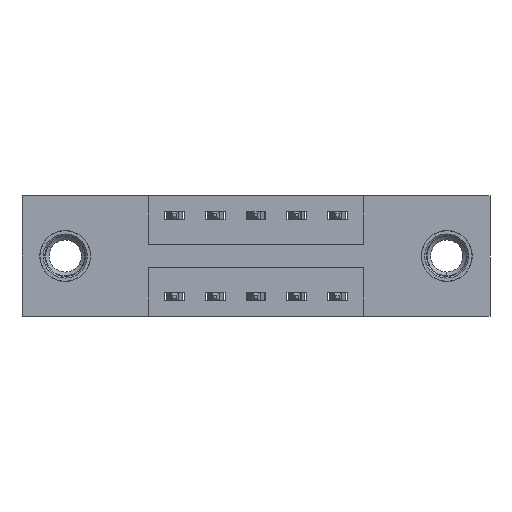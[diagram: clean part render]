
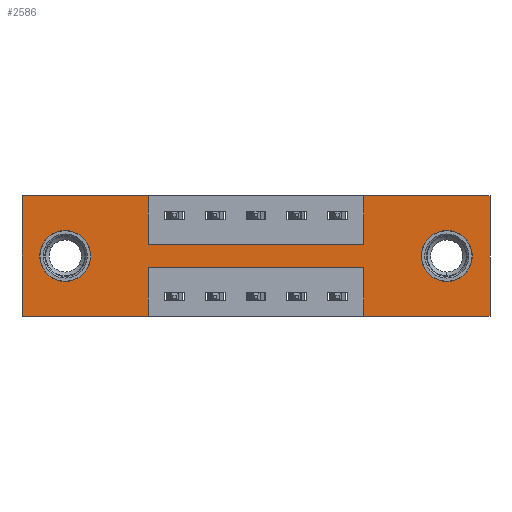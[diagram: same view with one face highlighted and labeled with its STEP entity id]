
A CAD part, front view. The second image highlights one B-rep face of the part: STEP entity #2586.
In plain terms, the highlighted planar face has unit normal (0, -1, 0).
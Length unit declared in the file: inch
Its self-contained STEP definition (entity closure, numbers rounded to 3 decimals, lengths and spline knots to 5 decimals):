
#34 = ORIENTED_EDGE ( 'NONE', *, *, #7145, .F. ) ;
#138 = CARTESIAN_POINT ( 'NONE',  ( 1.0475, 0., -0.37 ) ) ;
#144 = EDGE_CURVE ( 'NONE', #8442, #2010, #308, .T. ) ;
#201 = LINE ( 'NONE', #477, #5278 ) ;
#285 = AXIS2_PLACEMENT_3D ( 'NONE', #3052, #1589, #2337 ) ;
#308 = LINE ( 'NONE', #1299, #7852 ) ;
#352 = VECTOR ( 'NONE', #3183, 39.37008 ) ;
#371 = CARTESIAN_POINT ( 'NONE',  ( 1.0475, 0., 0. ) ) ;
#477 = CARTESIAN_POINT ( 'NONE',  ( 0.3875, 0., -0.22 ) ) ;
#523 = CARTESIAN_POINT ( 'NONE',  ( 0., 0., 0. ) ) ;
#541 = ORIENTED_EDGE ( 'NONE', *, *, #144, .F. ) ;
#603 = EDGE_CURVE ( 'NONE', #8182, #4735, #4690, .T. ) ;
#714 = EDGE_CURVE ( 'NONE', #3552, #2318, #6681, .T. ) ;
#733 = DIRECTION ( 'NONE',  ( 0., 1., 0. ) ) ;
#803 = CARTESIAN_POINT ( 'NONE',  ( 1.3025, 0., -0.185 ) ) ;
#824 = ORIENTED_EDGE ( 'NONE', *, *, #1951, .F. ) ;
#842 = ORIENTED_EDGE ( 'NONE', *, *, #8638, .F. ) ;
#930 = CARTESIAN_POINT ( 'NONE',  ( 0.1325, 0., -0.107 ) ) ;
#1009 = AXIS2_PLACEMENT_3D ( 'NONE', #3144, #6067, #7559 ) ;
#1018 = CARTESIAN_POINT ( 'NONE',  ( 1.3025, 0., -0.107 ) ) ;
#1029 = CARTESIAN_POINT ( 'NONE',  ( 0.3875, 0., -0.37 ) ) ;
#1113 = VECTOR ( 'NONE', #6441, 39.37008 ) ;
#1117 = ORIENTED_EDGE ( 'NONE', *, *, #6312, .F. ) ;
#1160 = VERTEX_POINT ( 'NONE', #3002 ) ;
#1279 = CARTESIAN_POINT ( 'NONE',  ( 0.3875, 0., 0. ) ) ;
#1299 = CARTESIAN_POINT ( 'NONE',  ( 0., 0., -0.37 ) ) ;
#1453 = CIRCLE ( 'NONE', #1009, 0.078 ) ;
#1497 = CARTESIAN_POINT ( 'NONE',  ( 0., 0., 0. ) ) ;
#1589 = DIRECTION ( 'NONE',  ( 0., -1., 0. ) ) ;
#1654 = ORIENTED_EDGE ( 'NONE', *, *, #3558, .F. ) ;
#1706 = EDGE_LOOP ( 'NONE', ( #4394, #842, #2827, #1654, #824, #2341, #4099, #1117, #34, #1812, #7414, #541 ) ) ;
#1734 = EDGE_CURVE ( 'NONE', #4735, #8182, #1453, .T. ) ;
#1739 = VERTEX_POINT ( 'NONE', #2428 ) ;
#1812 = ORIENTED_EDGE ( 'NONE', *, *, #714, .F. ) ;
#1835 = DIRECTION ( 'NONE',  ( 0., 0., -1. ) ) ;
#1866 = DIRECTION ( 'NONE',  ( 0., 0., 1. ) ) ;
#1901 = DIRECTION ( 'NONE',  ( 1., 0., 0. ) ) ;
#1946 = DIRECTION ( 'NONE',  ( 0., 0., 1. ) ) ;
#1951 = EDGE_CURVE ( 'NONE', #2083, #1739, #7568, .T. ) ;
#2010 = VERTEX_POINT ( 'NONE', #6331 ) ;
#2067 = CARTESIAN_POINT ( 'NONE',  ( 0.1325, 0., -0.185 ) ) ;
#2083 = VERTEX_POINT ( 'NONE', #2838 ) ;
#2204 = EDGE_LOOP ( 'NONE', ( #6551, #8420 ) ) ;
#2233 = LINE ( 'NONE', #1029, #7518 ) ;
#2293 = CARTESIAN_POINT ( 'NONE',  ( 0.3875, 0., -0.37 ) ) ;
#2318 = VERTEX_POINT ( 'NONE', #3682 ) ;
#2337 = DIRECTION ( 'NONE',  ( 0., 0., -1. ) ) ;
#2341 = ORIENTED_EDGE ( 'NONE', *, *, #3875, .F. ) ;
#2377 = LINE ( 'NONE', #4600, #352 ) ;
#2428 = CARTESIAN_POINT ( 'NONE',  ( 1.435, 0., -0.37 ) ) ;
#2482 = ORIENTED_EDGE ( 'NONE', *, *, #1734, .T. ) ;
#2554 = CARTESIAN_POINT ( 'NONE',  ( 0., 0., 0. ) ) ;
#2586 = ADVANCED_FACE ( 'NONE', ( #3332, #8987, #6343 ), #8069, .T. ) ;
#2632 = LINE ( 'NONE', #1497, #1113 ) ;
#2732 = VECTOR ( 'NONE', #4828, 39.37008 ) ;
#2827 = ORIENTED_EDGE ( 'NONE', *, *, #5557, .F. ) ;
#2838 = CARTESIAN_POINT ( 'NONE',  ( 1.435, 0., 0. ) ) ;
#2844 = DIRECTION ( 'NONE',  ( -1., 0., 0. ) ) ;
#3002 = CARTESIAN_POINT ( 'NONE',  ( 0.3875, 0., -0.15 ) ) ;
#3052 = CARTESIAN_POINT ( 'NONE',  ( 0., 0., -0.37 ) ) ;
#3058 = CARTESIAN_POINT ( 'NONE',  ( 1.0475, 0., -0.22 ) ) ;
#3084 = DIRECTION ( 'NONE',  ( -1., 0., 0. ) ) ;
#3144 = CARTESIAN_POINT ( 'NONE',  ( 1.3025, 0., -0.185 ) ) ;
#3183 = DIRECTION ( 'NONE',  ( 1., 0., 0. ) ) ;
#3316 = CARTESIAN_POINT ( 'NONE',  ( 0., 0., 0. ) ) ;
#3326 = AXIS2_PLACEMENT_3D ( 'NONE', #803, #733, #5906 ) ;
#3332 = FACE_BOUND ( 'NONE', #8821, .T. ) ;
#3365 = VECTOR ( 'NONE', #1946, 39.37008 ) ;
#3400 = EDGE_CURVE ( 'NONE', #2010, #3552, #3586, .T. ) ;
#3552 = VERTEX_POINT ( 'NONE', #523 ) ;
#3558 = EDGE_CURVE ( 'NONE', #1739, #6993, #7531, .T. ) ;
#3564 = DIRECTION ( 'NONE',  ( 0., 0., -1. ) ) ;
#3578 = CARTESIAN_POINT ( 'NONE',  ( 0.1325, 0., -0.263 ) ) ;
#3586 = LINE ( 'NONE', #3316, #3365 ) ;
#3637 = VERTEX_POINT ( 'NONE', #3725 ) ;
#3676 = DIRECTION ( 'NONE',  ( 0., 0., 1. ) ) ;
#3682 = CARTESIAN_POINT ( 'NONE',  ( 0.3875, 0., 0. ) ) ;
#3725 = CARTESIAN_POINT ( 'NONE',  ( 1.0475, 0., -0.15 ) ) ;
#3872 = VECTOR ( 'NONE', #1901, 39.37008 ) ;
#3875 = EDGE_CURVE ( 'NONE', #8345, #2083, #2632, .T. ) ;
#3980 = LINE ( 'NONE', #371, #8834 ) ;
#4028 = CARTESIAN_POINT ( 'NONE',  ( 1.435, 0., 0. ) ) ;
#4099 = ORIENTED_EDGE ( 'NONE', *, *, #4216, .F. ) ;
#4163 = CIRCLE ( 'NONE', #7188, 0.078 ) ;
#4216 = EDGE_CURVE ( 'NONE', #3637, #8345, #3980, .T. ) ;
#4343 = CIRCLE ( 'NONE', #4488, 0.078 ) ;
#4394 = ORIENTED_EDGE ( 'NONE', *, *, #9007, .F. ) ;
#4488 = AXIS2_PLACEMENT_3D ( 'NONE', #8062, #8000, #3676 ) ;
#4600 = CARTESIAN_POINT ( 'NONE',  ( 0.3875, 0., -0.15 ) ) ;
#4690 = CIRCLE ( 'NONE', #3326, 0.078 ) ;
#4735 = VERTEX_POINT ( 'NONE', #1018 ) ;
#4800 = CARTESIAN_POINT ( 'NONE',  ( 1.0475, 0., -0.37 ) ) ;
#4828 = DIRECTION ( 'NONE',  ( 0., 0., -1. ) ) ;
#5278 = VECTOR ( 'NONE', #9164, 39.37008 ) ;
#5557 = EDGE_CURVE ( 'NONE', #6993, #8505, #7197, .T. ) ;
#5684 = DIRECTION ( 'NONE',  ( 0., 0., 1. ) ) ;
#5872 = LINE ( 'NONE', #1279, #8563 ) ;
#5906 = DIRECTION ( 'NONE',  ( 0., 0., -1. ) ) ;
#5945 = VECTOR ( 'NONE', #3084, 39.37008 ) ;
#6067 = DIRECTION ( 'NONE',  ( 0., 1., 0. ) ) ;
#6075 = CARTESIAN_POINT ( 'NONE',  ( 0., 0., -0.37 ) ) ;
#6312 = EDGE_CURVE ( 'NONE', #1160, #3637, #2377, .T. ) ;
#6331 = CARTESIAN_POINT ( 'NONE',  ( 0., 0., -0.37 ) ) ;
#6343 = FACE_OUTER_BOUND ( 'NONE', #1706, .T. ) ;
#6351 = ORIENTED_EDGE ( 'NONE', *, *, #603, .T. ) ;
#6370 = DIRECTION ( 'NONE',  ( 0., 1., 0. ) ) ;
#6379 = CARTESIAN_POINT ( 'NONE',  ( 1.0475, 0., 0. ) ) ;
#6435 = EDGE_CURVE ( 'NONE', #7202, #9471, #4163, .T. ) ;
#6441 = DIRECTION ( 'NONE',  ( 1., 0., 0. ) ) ;
#6551 = ORIENTED_EDGE ( 'NONE', *, *, #6435, .T. ) ;
#6681 = LINE ( 'NONE', #2554, #3872 ) ;
#6816 = CARTESIAN_POINT ( 'NONE',  ( 0.3875, 0., -0.22 ) ) ;
#6993 = VERTEX_POINT ( 'NONE', #138 ) ;
#6997 = DIRECTION ( 'NONE',  ( 0., 0., 1. ) ) ;
#7145 = EDGE_CURVE ( 'NONE', #2318, #1160, #5872, .T. ) ;
#7188 = AXIS2_PLACEMENT_3D ( 'NONE', #2067, #6370, #5684 ) ;
#7197 = LINE ( 'NONE', #4800, #8885 ) ;
#7202 = VERTEX_POINT ( 'NONE', #930 ) ;
#7414 = ORIENTED_EDGE ( 'NONE', *, *, #3400, .F. ) ;
#7518 = VECTOR ( 'NONE', #1835, 39.37008 ) ;
#7531 = LINE ( 'NONE', #6075, #5945 ) ;
#7559 = DIRECTION ( 'NONE',  ( 0., 0., -1. ) ) ;
#7568 = LINE ( 'NONE', #4028, #2732 ) ;
#7852 = VECTOR ( 'NONE', #2844, 39.37008 ) ;
#8000 = DIRECTION ( 'NONE',  ( 0., 1., 0. ) ) ;
#8062 = CARTESIAN_POINT ( 'NONE',  ( 0.1325, 0., -0.185 ) ) ;
#8069 = PLANE ( 'NONE',  #285 ) ;
#8132 = VERTEX_POINT ( 'NONE', #6816 ) ;
#8182 = VERTEX_POINT ( 'NONE', #9218 ) ;
#8345 = VERTEX_POINT ( 'NONE', #6379 ) ;
#8420 = ORIENTED_EDGE ( 'NONE', *, *, #9255, .T. ) ;
#8442 = VERTEX_POINT ( 'NONE', #2293 ) ;
#8505 = VERTEX_POINT ( 'NONE', #3058 ) ;
#8563 = VECTOR ( 'NONE', #3564, 39.37008 ) ;
#8638 = EDGE_CURVE ( 'NONE', #8505, #8132, #201, .T. ) ;
#8821 = EDGE_LOOP ( 'NONE', ( #2482, #6351 ) ) ;
#8834 = VECTOR ( 'NONE', #6997, 39.37008 ) ;
#8885 = VECTOR ( 'NONE', #1866, 39.37008 ) ;
#8987 = FACE_BOUND ( 'NONE', #2204, .T. ) ;
#9007 = EDGE_CURVE ( 'NONE', #8132, #8442, #2233, .T. ) ;
#9164 = DIRECTION ( 'NONE',  ( -1., 0., 0. ) ) ;
#9218 = CARTESIAN_POINT ( 'NONE',  ( 1.3025, 0., -0.263 ) ) ;
#9255 = EDGE_CURVE ( 'NONE', #9471, #7202, #4343, .T. ) ;
#9471 = VERTEX_POINT ( 'NONE', #3578 ) ;
